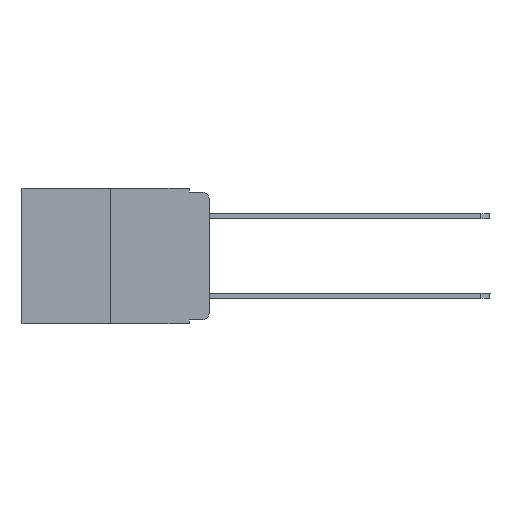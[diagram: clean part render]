
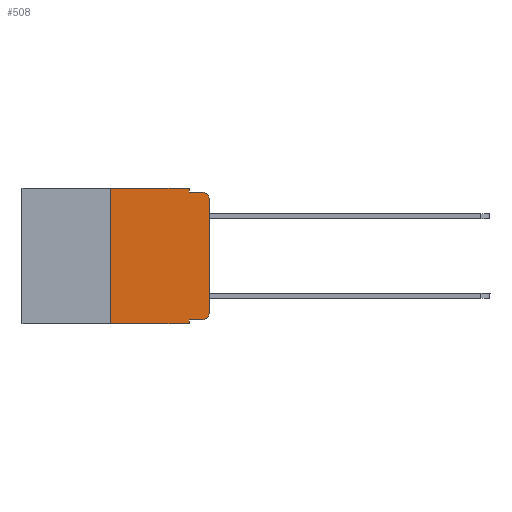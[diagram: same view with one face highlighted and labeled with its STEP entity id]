
A CAD part, left-side view. The second image highlights one B-rep face of the part: STEP entity #508.
In plain terms, the highlighted planar face has unit normal (-1, 0, 0).
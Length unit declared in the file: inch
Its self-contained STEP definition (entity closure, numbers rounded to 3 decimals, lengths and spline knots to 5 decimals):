
#251 = VERTEX_POINT ( 'NONE', #14051 ) ;
#508 = ADVANCED_FACE ( 'NONE', ( #7547 ), #6022, .F. ) ;
#830 = LINE ( 'NONE', #10747, #14079 ) ;
#1059 = CARTESIAN_POINT ( 'NONE',  ( 0., 0.02, -0.03 ) ) ;
#1146 = VERTEX_POINT ( 'NONE', #1661 ) ;
#1194 = ORIENTED_EDGE ( 'NONE', *, *, #14596, .T. ) ;
#1661 = CARTESIAN_POINT ( 'NONE',  ( 0., 0.051, -0.333 ) ) ;
#1724 = CIRCLE ( 'NONE', #5160, 0.02 ) ;
#1802 = EDGE_CURVE ( 'NONE', #251, #13666, #17583, .T. ) ;
#2064 = DIRECTION ( 'NONE',  ( 0., 0., -1. ) ) ;
#2241 = VECTOR ( 'NONE', #10047, 39.37008 ) ;
#2250 = ORIENTED_EDGE ( 'NONE', *, *, #2482, .F. ) ;
#2482 = EDGE_CURVE ( 'NONE', #1146, #15117, #8782, .T. ) ;
#3018 = VECTOR ( 'NONE', #15737, 39.37008 ) ;
#3207 = ORIENTED_EDGE ( 'NONE', *, *, #3906, .F. ) ;
#3267 = ORIENTED_EDGE ( 'NONE', *, *, #15665, .F. ) ;
#3906 = EDGE_CURVE ( 'NONE', #4953, #251, #6166, .T. ) ;
#3936 = ORIENTED_EDGE ( 'NONE', *, *, #1802, .F. ) ;
#4358 = CIRCLE ( 'NONE', #15308, 0.02 ) ;
#4525 = CARTESIAN_POINT ( 'NONE',  ( 0., 0.051, -0.343 ) ) ;
#4646 = ORIENTED_EDGE ( 'NONE', *, *, #13899, .T. ) ;
#4733 = CARTESIAN_POINT ( 'NONE',  ( 0., 0.051, 0. ) ) ;
#4735 = CARTESIAN_POINT ( 'NONE',  ( 0., 0.25, 0. ) ) ;
#4953 = VERTEX_POINT ( 'NONE', #15209 ) ;
#4971 = VERTEX_POINT ( 'NONE', #15970 ) ;
#5160 = AXIS2_PLACEMENT_3D ( 'NONE', #1059, #13591, #13323 ) ;
#5236 = VERTEX_POINT ( 'NONE', #13030 ) ;
#5377 = DIRECTION ( 'NONE',  ( 0., 0., -1. ) ) ;
#5949 = CARTESIAN_POINT ( 'NONE',  ( 0., 0., -0.03 ) ) ;
#6022 = PLANE ( 'NONE',  #15123 ) ;
#6155 = LINE ( 'NONE', #14379, #2241 ) ;
#6166 = LINE ( 'NONE', #4735, #3018 ) ;
#6446 = CARTESIAN_POINT ( 'NONE',  ( 0., 0.02, -0.313 ) ) ;
#6622 = DIRECTION ( 'NONE',  ( 0., -1., 0. ) ) ;
#6647 = DIRECTION ( 'NONE',  ( 0., -1., 0. ) ) ;
#6909 = ORIENTED_EDGE ( 'NONE', *, *, #13557, .T. ) ;
#7547 = FACE_OUTER_BOUND ( 'NONE', #14611, .T. ) ;
#7658 = CARTESIAN_POINT ( 'NONE',  ( 0., 0.02, -0.01 ) ) ;
#8782 = LINE ( 'NONE', #4733, #14465 ) ;
#8821 = LINE ( 'NONE', #15688, #9200 ) ;
#9200 = VECTOR ( 'NONE', #6622, 39.37008 ) ;
#9210 = CARTESIAN_POINT ( 'NONE',  ( 0., 0.051, 0. ) ) ;
#9279 = CARTESIAN_POINT ( 'NONE',  ( 0., 0.473, 0. ) ) ;
#9465 = ORIENTED_EDGE ( 'NONE', *, *, #15578, .T. ) ;
#9516 = VERTEX_POINT ( 'NONE', #5949 ) ;
#9799 = VECTOR ( 'NONE', #12831, 39.37008 ) ;
#10047 = DIRECTION ( 'NONE',  ( 0., 0., -1. ) ) ;
#10241 = EDGE_CURVE ( 'NONE', #13666, #16016, #6155, .T. ) ;
#10747 = CARTESIAN_POINT ( 'NONE',  ( 0., 0.473, -0.343 ) ) ;
#10858 = VERTEX_POINT ( 'NONE', #7658 ) ;
#10929 = VECTOR ( 'NONE', #11442, 39.37008 ) ;
#11318 = CARTESIAN_POINT ( 'NONE',  ( 0., 0.051, -0.01 ) ) ;
#11354 = CARTESIAN_POINT ( 'NONE',  ( 0., 0., 0. ) ) ;
#11442 = DIRECTION ( 'NONE',  ( 0., 0., 1. ) ) ;
#11495 = DIRECTION ( 'NONE',  ( 0., 0., -1. ) ) ;
#11528 = CARTESIAN_POINT ( 'NONE',  ( 0., 0.473, 0. ) ) ;
#12703 = LINE ( 'NONE', #11354, #10929 ) ;
#12831 = DIRECTION ( 'NONE',  ( 0., -1., 0. ) ) ;
#13030 = CARTESIAN_POINT ( 'NONE',  ( 0., 0.02, -0.333 ) ) ;
#13174 = DIRECTION ( 'NONE',  ( 0., -1., 0. ) ) ;
#13323 = DIRECTION ( 'NONE',  ( 0., 0., -1. ) ) ;
#13557 = EDGE_CURVE ( 'NONE', #4953, #15117, #830, .T. ) ;
#13591 = DIRECTION ( 'NONE',  ( -1., 0., 0. ) ) ;
#13666 = VERTEX_POINT ( 'NONE', #9210 ) ;
#13899 = EDGE_CURVE ( 'NONE', #9516, #10858, #1724, .T. ) ;
#14051 = CARTESIAN_POINT ( 'NONE',  ( 0., 0.25, 0. ) ) ;
#14079 = VECTOR ( 'NONE', #13174, 39.37008 ) ;
#14207 = ORIENTED_EDGE ( 'NONE', *, *, #17516, .T. ) ;
#14278 = ORIENTED_EDGE ( 'NONE', *, *, #10241, .F. ) ;
#14379 = CARTESIAN_POINT ( 'NONE',  ( 0., 0.051, 0. ) ) ;
#14465 = VECTOR ( 'NONE', #11495, 39.37008 ) ;
#14500 = DIRECTION ( 'NONE',  ( -1., 0., 0. ) ) ;
#14596 = EDGE_CURVE ( 'NONE', #1146, #5236, #17085, .T. ) ;
#14611 = EDGE_LOOP ( 'NONE', ( #9465, #4646, #3267, #14278, #3936, #3207, #6909, #2250, #1194, #14207 ) ) ;
#15117 = VERTEX_POINT ( 'NONE', #4525 ) ;
#15123 = AXIS2_PLACEMENT_3D ( 'NONE', #11528, #17033, #5377 ) ;
#15209 = CARTESIAN_POINT ( 'NONE',  ( 0., 0.25, -0.343 ) ) ;
#15308 = AXIS2_PLACEMENT_3D ( 'NONE', #6446, #14500, #2064 ) ;
#15578 = EDGE_CURVE ( 'NONE', #4971, #9516, #12703, .T. ) ;
#15646 = CARTESIAN_POINT ( 'NONE',  ( 0., 0.051, -0.333 ) ) ;
#15665 = EDGE_CURVE ( 'NONE', #16016, #10858, #8821, .T. ) ;
#15688 = CARTESIAN_POINT ( 'NONE',  ( 0., 0.051, -0.01 ) ) ;
#15737 = DIRECTION ( 'NONE',  ( 0., 0., 1. ) ) ;
#15970 = CARTESIAN_POINT ( 'NONE',  ( 0., 0., -0.313 ) ) ;
#16016 = VERTEX_POINT ( 'NONE', #11318 ) ;
#16037 = VECTOR ( 'NONE', #6647, 39.37008 ) ;
#17033 = DIRECTION ( 'NONE',  ( 1., 0., 0. ) ) ;
#17085 = LINE ( 'NONE', #15646, #9799 ) ;
#17516 = EDGE_CURVE ( 'NONE', #5236, #4971, #4358, .T. ) ;
#17583 = LINE ( 'NONE', #9279, #16037 ) ;
